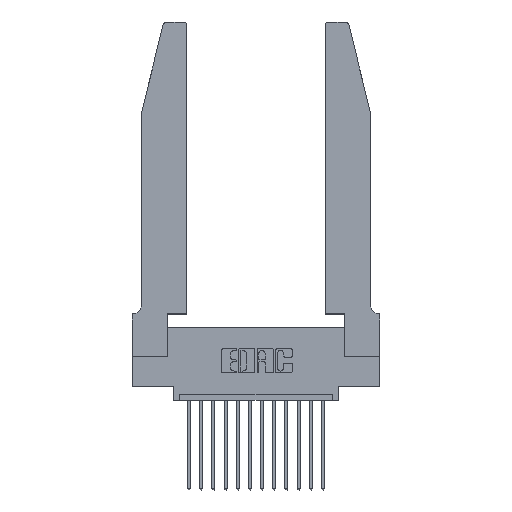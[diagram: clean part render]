
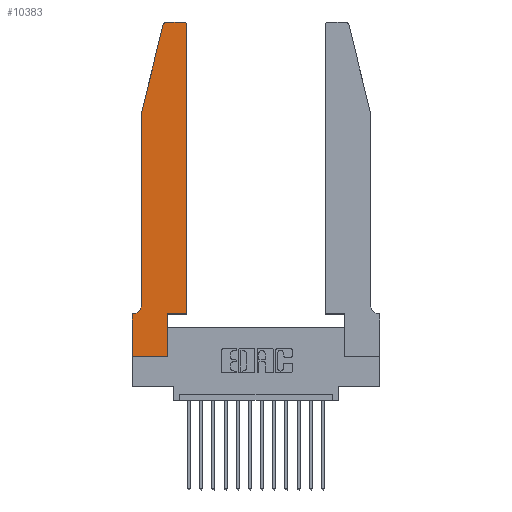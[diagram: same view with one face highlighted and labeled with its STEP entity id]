
A CAD part, top view. The second image highlights one B-rep face of the part: STEP entity #10383.
In plain terms, the highlighted planar face has unit normal (0, 0, 1).
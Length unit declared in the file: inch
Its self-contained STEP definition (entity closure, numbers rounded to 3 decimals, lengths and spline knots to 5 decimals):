
#111 = VERTEX_POINT ( 'NONE', #2508 ) ;
#155 = VECTOR ( 'NONE', #12949, 39.37008 ) ;
#169 = AXIS2_PLACEMENT_3D ( 'NONE', #17359, #6286, #10546 ) ;
#174 = DIRECTION ( 'NONE',  ( -0.239, -0.971, 0. ) ) ;
#300 = CARTESIAN_POINT ( 'NONE',  ( 0.0755, 0.35, 0.37 ) ) ;
#1034 = LINE ( 'NONE', #9974, #12075 ) ;
#1324 = DIRECTION ( 'NONE',  ( 1., 0., 0. ) ) ;
#1661 = EDGE_CURVE ( 'NONE', #111, #15674, #5357, .T. ) ;
#1849 = LINE ( 'NONE', #12741, #6586 ) ;
#1850 = CARTESIAN_POINT ( 'NONE',  ( 0.4505, 2.72, 0.37 ) ) ;
#2180 = DIRECTION ( 'NONE',  ( 1., 0., 0. ) ) ;
#2184 = EDGE_CURVE ( 'NONE', #2569, #3996, #3384, .T. ) ;
#2295 = EDGE_CURVE ( 'NONE', #14558, #111, #1034, .T. ) ;
#2327 = VERTEX_POINT ( 'NONE', #17452 ) ;
#2355 = LINE ( 'NONE', #14518, #10577 ) ;
#2508 = CARTESIAN_POINT ( 'NONE',  ( 0.284, 2.75, 0.37 ) ) ;
#2569 = VERTEX_POINT ( 'NONE', #15278 ) ;
#2711 = ORIENTED_EDGE ( 'NONE', *, *, #17694, .T. ) ;
#2836 = DIRECTION ( 'NONE',  ( 0., 0., 1. ) ) ;
#3384 = LINE ( 'NONE', #300, #155 ) ;
#3535 = VECTOR ( 'NONE', #15970, 39.37008 ) ;
#3901 = VECTOR ( 'NONE', #4925, 39.37008 ) ;
#3996 = VERTEX_POINT ( 'NONE', #11888 ) ;
#4168 = EDGE_CURVE ( 'NONE', #7372, #5951, #1849, .T. ) ;
#4504 = ORIENTED_EDGE ( 'NONE', *, *, #2295, .T. ) ;
#4557 = CIRCLE ( 'NONE', #7099, 0.03 ) ;
#4587 = VERTEX_POINT ( 'NONE', #13733 ) ;
#4605 = FACE_OUTER_BOUND ( 'NONE', #5626, .T. ) ;
#4808 = VECTOR ( 'NONE', #174, 39.37008 ) ;
#4853 = CIRCLE ( 'NONE', #169, 0.07 ) ;
#4925 = DIRECTION ( 'NONE',  ( 0., -1., 0. ) ) ;
#5357 = CIRCLE ( 'NONE', #12530, 0.03 ) ;
#5362 = DIRECTION ( 'NONE',  ( 1., 0., 0. ) ) ;
#5570 = ORIENTED_EDGE ( 'NONE', *, *, #9144, .T. ) ;
#5595 = DIRECTION ( 'NONE',  ( 1., 0., 0. ) ) ;
#5622 = ORIENTED_EDGE ( 'NONE', *, *, #16850, .T. ) ;
#5626 = EDGE_LOOP ( 'NONE', ( #4504, #15443, #15230, #8802, #5622, #16259, #17524, #6972, #5570, #2711, #11721, #11283 ) ) ;
#5851 = CARTESIAN_POINT ( 'NONE',  ( 0.4205, 2.75, 0.37 ) ) ;
#5951 = VERTEX_POINT ( 'NONE', #1850 ) ;
#6286 = DIRECTION ( 'NONE',  ( 0., 0., -1. ) ) ;
#6320 = VECTOR ( 'NONE', #5362, 39.37008 ) ;
#6331 = VERTEX_POINT ( 'NONE', #6855 ) ;
#6586 = VECTOR ( 'NONE', #9925, 39.37008 ) ;
#6739 = EDGE_CURVE ( 'NONE', #5951, #14558, #4557, .T. ) ;
#6787 = CARTESIAN_POINT ( 'NONE',  ( 0.0755, 2., 0.37 ) ) ;
#6855 = CARTESIAN_POINT ( 'NONE',  ( 0.2865, 0.35, 0.37 ) ) ;
#6972 = ORIENTED_EDGE ( 'NONE', *, *, #11736, .T. ) ;
#7099 = AXIS2_PLACEMENT_3D ( 'NONE', #8236, #8355, #1324 ) ;
#7326 = LINE ( 'NONE', #8050, #13863 ) ;
#7328 = VERTEX_POINT ( 'NONE', #10771 ) ;
#7372 = VERTEX_POINT ( 'NONE', #9326 ) ;
#7895 = CARTESIAN_POINT ( 'NONE',  ( 0.0755, 2., 0.37 ) ) ;
#8050 = CARTESIAN_POINT ( 'NONE',  ( 0., 0., 0.37 ) ) ;
#8236 = CARTESIAN_POINT ( 'NONE',  ( 0.4205, 2.72, 0.37 ) ) ;
#8320 = VERTEX_POINT ( 'NONE', #7895 ) ;
#8355 = DIRECTION ( 'NONE',  ( 0., 0., 1. ) ) ;
#8471 = LINE ( 'NONE', #6787, #4808 ) ;
#8802 = ORIENTED_EDGE ( 'NONE', *, *, #12957, .T. ) ;
#9093 = CARTESIAN_POINT ( 'NONE',  ( 0., 0., 0.37 ) ) ;
#9144 = EDGE_CURVE ( 'NONE', #7328, #6331, #15480, .T. ) ;
#9326 = CARTESIAN_POINT ( 'NONE',  ( 0.4505, 0.35, 0.37 ) ) ;
#9896 = CARTESIAN_POINT ( 'NONE',  ( 0., 0.35, 0.37 ) ) ;
#9925 = DIRECTION ( 'NONE',  ( 0., 1., 0. ) ) ;
#9974 = CARTESIAN_POINT ( 'NONE',  ( 0.2605, 2.75, 0.37 ) ) ;
#10314 = EDGE_CURVE ( 'NONE', #15674, #8320, #8471, .T. ) ;
#10383 = ADVANCED_FACE ( 'NONE', ( #4605 ), #14026, .T. ) ;
#10462 = DIRECTION ( 'NONE',  ( 0., 0., 1. ) ) ;
#10546 = DIRECTION ( 'NONE',  ( -1., 0., 0. ) ) ;
#10577 = VECTOR ( 'NONE', #15814, 39.37008 ) ;
#10771 = CARTESIAN_POINT ( 'NONE',  ( 0.2865, 0., 0.37 ) ) ;
#11283 = ORIENTED_EDGE ( 'NONE', *, *, #6739, .T. ) ;
#11578 = EDGE_CURVE ( 'NONE', #3996, #2327, #14290, .T. ) ;
#11693 = CARTESIAN_POINT ( 'NONE',  ( 0.284, 2.72, 0.37 ) ) ;
#11721 = ORIENTED_EDGE ( 'NONE', *, *, #4168, .T. ) ;
#11736 = EDGE_CURVE ( 'NONE', #2327, #7328, #7326, .T. ) ;
#11857 = DIRECTION ( 'NONE',  ( -1., 0., 0. ) ) ;
#11888 = CARTESIAN_POINT ( 'NONE',  ( 0., 0.35, 0.37 ) ) ;
#12075 = VECTOR ( 'NONE', #11857, 39.37008 ) ;
#12530 = AXIS2_PLACEMENT_3D ( 'NONE', #11693, #10462, #2180 ) ;
#12741 = CARTESIAN_POINT ( 'NONE',  ( 0.4505, 0.35, 0.37 ) ) ;
#12949 = DIRECTION ( 'NONE',  ( -1., 0., 0. ) ) ;
#12957 = EDGE_CURVE ( 'NONE', #8320, #4587, #2355, .T. ) ;
#13109 = CARTESIAN_POINT ( 'NONE',  ( 0.2865, 0.35, 0.37 ) ) ;
#13477 = LINE ( 'NONE', #16477, #6320 ) ;
#13733 = CARTESIAN_POINT ( 'NONE',  ( 0.0755, 0.42, 0.37 ) ) ;
#13863 = VECTOR ( 'NONE', #14736, 39.37008 ) ;
#14026 = PLANE ( 'NONE',  #14133 ) ;
#14133 = AXIS2_PLACEMENT_3D ( 'NONE', #9896, #2836, #5595 ) ;
#14290 = LINE ( 'NONE', #9093, #3901 ) ;
#14518 = CARTESIAN_POINT ( 'NONE',  ( 0.0755, 2., 0.37 ) ) ;
#14558 = VERTEX_POINT ( 'NONE', #5851 ) ;
#14736 = DIRECTION ( 'NONE',  ( 1., 0., 0. ) ) ;
#15230 = ORIENTED_EDGE ( 'NONE', *, *, #10314, .T. ) ;
#15278 = CARTESIAN_POINT ( 'NONE',  ( 0.0055, 0.35, 0.37 ) ) ;
#15443 = ORIENTED_EDGE ( 'NONE', *, *, #1661, .T. ) ;
#15480 = LINE ( 'NONE', #13109, #3535 ) ;
#15674 = VERTEX_POINT ( 'NONE', #16216 ) ;
#15814 = DIRECTION ( 'NONE',  ( 0., -1., 0. ) ) ;
#15970 = DIRECTION ( 'NONE',  ( 0., 1., 0. ) ) ;
#16216 = CARTESIAN_POINT ( 'NONE',  ( 0.25487, 2.72718, 0.37 ) ) ;
#16259 = ORIENTED_EDGE ( 'NONE', *, *, #2184, .T. ) ;
#16477 = CARTESIAN_POINT ( 'NONE',  ( 0.4505, 0.35, 0.37 ) ) ;
#16850 = EDGE_CURVE ( 'NONE', #4587, #2569, #4853, .T. ) ;
#17359 = CARTESIAN_POINT ( 'NONE',  ( 0.0055, 0.42, 0.37 ) ) ;
#17452 = CARTESIAN_POINT ( 'NONE',  ( 0., 0., 0.37 ) ) ;
#17524 = ORIENTED_EDGE ( 'NONE', *, *, #11578, .T. ) ;
#17694 = EDGE_CURVE ( 'NONE', #6331, #7372, #13477, .T. ) ;
